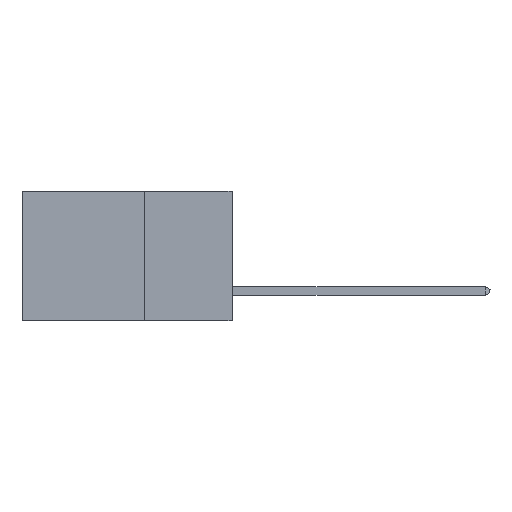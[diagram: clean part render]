
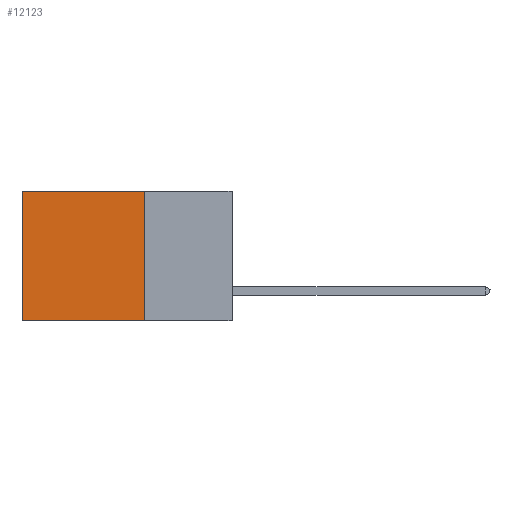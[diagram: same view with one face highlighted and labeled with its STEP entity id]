
A CAD part, left-side view. The second image highlights one B-rep face of the part: STEP entity #12123.
In plain terms, the highlighted planar face has unit normal (-1, 0, 0).
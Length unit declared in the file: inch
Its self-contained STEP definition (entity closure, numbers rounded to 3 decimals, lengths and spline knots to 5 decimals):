
#482 = VERTEX_POINT ( 'NONE', #12712 ) ;
#488 = EDGE_CURVE ( 'NONE', #482, #9259, #11345, .T. ) ;
#1522 = VERTEX_POINT ( 'NONE', #11933 ) ;
#1719 = PLANE ( 'NONE',  #6475 ) ;
#3341 = EDGE_CURVE ( 'NONE', #1522, #9259, #3462, .T. ) ;
#3462 = LINE ( 'NONE', #8364, #9952 ) ;
#3581 = LINE ( 'NONE', #8482, #4985 ) ;
#3979 = EDGE_LOOP ( 'NONE', ( #8264, #15438, #14369, #10058 ) ) ;
#4985 = VECTOR ( 'NONE', #7279, 39.37008 ) ;
#5086 = DIRECTION ( 'NONE',  ( 0., 1., 0. ) ) ;
#5347 = CARTESIAN_POINT ( 'NONE',  ( 0.2875, 0.25, 0. ) ) ;
#6475 = AXIS2_PLACEMENT_3D ( 'NONE', #8000, #12696, #10512 ) ;
#7205 = VECTOR ( 'NONE', #12629, 39.37008 ) ;
#7279 = DIRECTION ( 'NONE',  ( 0., 0., -1. ) ) ;
#7657 = LINE ( 'NONE', #12505, #13997 ) ;
#8000 = CARTESIAN_POINT ( 'NONE',  ( 0.2875, 0.25, 0. ) ) ;
#8101 = EDGE_CURVE ( 'NONE', #14613, #1522, #7657, .T. ) ;
#8127 = DIRECTION ( 'NONE',  ( 0., 0., -1. ) ) ;
#8264 = ORIENTED_EDGE ( 'NONE', *, *, #3341, .T. ) ;
#8300 = EDGE_CURVE ( 'NONE', #14613, #482, #3581, .T. ) ;
#8364 = CARTESIAN_POINT ( 'NONE',  ( 0.2875, 0.6, 0. ) ) ;
#8482 = CARTESIAN_POINT ( 'NONE',  ( 0.2875, 0.25, 0. ) ) ;
#9259 = VERTEX_POINT ( 'NONE', #14665 ) ;
#9952 = VECTOR ( 'NONE', #8127, 39.37008 ) ;
#10058 = ORIENTED_EDGE ( 'NONE', *, *, #8101, .T. ) ;
#10512 = DIRECTION ( 'NONE',  ( 0., 0., -1. ) ) ;
#11345 = LINE ( 'NONE', #11510, #7205 ) ;
#11510 = CARTESIAN_POINT ( 'NONE',  ( 0.2875, 0.25, -0.37 ) ) ;
#11933 = CARTESIAN_POINT ( 'NONE',  ( 0.2875, 0.6, 0. ) ) ;
#12123 = ADVANCED_FACE ( 'NONE', ( #13900 ), #1719, .F. ) ;
#12505 = CARTESIAN_POINT ( 'NONE',  ( 0.2875, 0.25, 0. ) ) ;
#12629 = DIRECTION ( 'NONE',  ( 0., 1., 0. ) ) ;
#12696 = DIRECTION ( 'NONE',  ( 1., 0., 0. ) ) ;
#12712 = CARTESIAN_POINT ( 'NONE',  ( 0.2875, 0.25, -0.37 ) ) ;
#13900 = FACE_OUTER_BOUND ( 'NONE', #3979, .T. ) ;
#13997 = VECTOR ( 'NONE', #5086, 39.37008 ) ;
#14369 = ORIENTED_EDGE ( 'NONE', *, *, #8300, .F. ) ;
#14613 = VERTEX_POINT ( 'NONE', #5347 ) ;
#14665 = CARTESIAN_POINT ( 'NONE',  ( 0.2875, 0.6, -0.37 ) ) ;
#15438 = ORIENTED_EDGE ( 'NONE', *, *, #488, .F. ) ;
